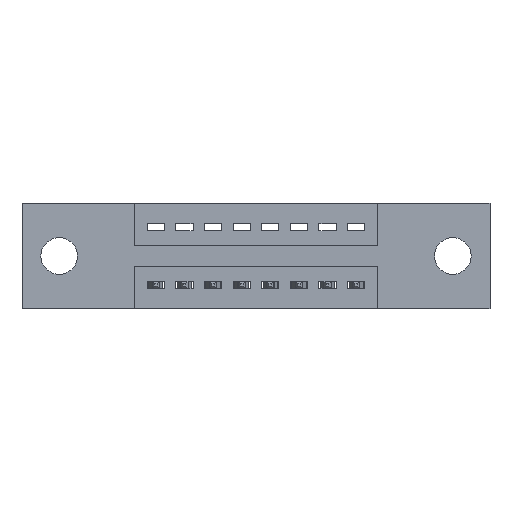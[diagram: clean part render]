
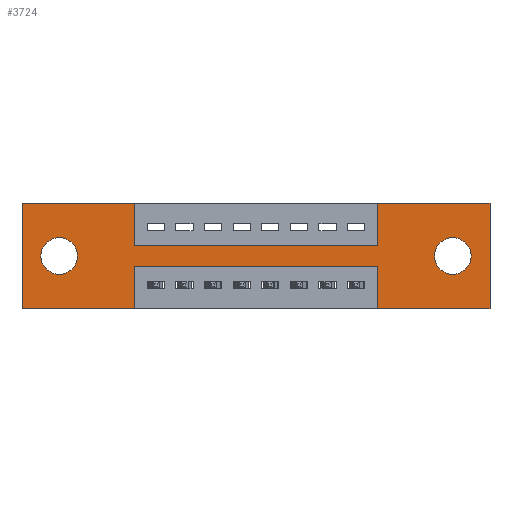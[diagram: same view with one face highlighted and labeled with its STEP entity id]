
A CAD part, front view. The second image highlights one B-rep face of the part: STEP entity #3724.
In plain terms, the highlighted planar face has unit normal (0, -1, 0).
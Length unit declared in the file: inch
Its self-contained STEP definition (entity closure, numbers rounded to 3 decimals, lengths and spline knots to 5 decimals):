
#4 = EDGE_LOOP ( 'NONE', ( #10293, #9271, #5013, #3844, #3061, #8803, #9520, #10448, #2262, #5152, #9273, #4067 ) ) ;
#35 = CIRCLE ( 'NONE', #8697, 0.064 ) ;
#240 = VECTOR ( 'NONE', #6881, 39.37008 ) ;
#347 = CARTESIAN_POINT ( 'NONE',  ( 0.3925, 0., -0.22 ) ) ;
#431 = EDGE_CURVE ( 'NONE', #10010, #1811, #8171, .T. ) ;
#432 = VECTOR ( 'NONE', #6179, 39.37008 ) ;
#490 = DIRECTION ( 'NONE',  ( 0., 0., -1. ) ) ;
#579 = EDGE_LOOP ( 'NONE', ( #4514, #2880 ) ) ;
#806 = CARTESIAN_POINT ( 'NONE',  ( 1.2425, 0., -0.37 ) ) ;
#995 = DIRECTION ( 'NONE',  ( 0., 1., 0. ) ) ;
#1017 = VECTOR ( 'NONE', #2011, 39.37008 ) ;
#1083 = VECTOR ( 'NONE', #9012, 39.37008 ) ;
#1107 = LINE ( 'NONE', #1482, #8126 ) ;
#1212 = VERTEX_POINT ( 'NONE', #10197 ) ;
#1329 = EDGE_CURVE ( 'NONE', #3986, #3708, #7113, .T. ) ;
#1361 = VERTEX_POINT ( 'NONE', #6587 ) ;
#1482 = CARTESIAN_POINT ( 'NONE',  ( 0.3925, 0., -0.37 ) ) ;
#1505 = CARTESIAN_POINT ( 'NONE',  ( 0.3925, 0., 0. ) ) ;
#1555 = CARTESIAN_POINT ( 'NONE',  ( 0.3925, 0., -0.22 ) ) ;
#1620 = CARTESIAN_POINT ( 'NONE',  ( 0., 0., 0. ) ) ;
#1656 = DIRECTION ( 'NONE',  ( 0., 0., 1. ) ) ;
#1811 = VERTEX_POINT ( 'NONE', #9409 ) ;
#1822 = EDGE_CURVE ( 'NONE', #7201, #1212, #8903, .T. ) ;
#1976 = CARTESIAN_POINT ( 'NONE',  ( 1.635, 0., 0. ) ) ;
#2011 = DIRECTION ( 'NONE',  ( 0., 0., -1. ) ) ;
#2190 = VECTOR ( 'NONE', #10179, 39.37008 ) ;
#2245 = CARTESIAN_POINT ( 'NONE',  ( 0.3925, 0., -0.15 ) ) ;
#2262 = ORIENTED_EDGE ( 'NONE', *, *, #7034, .F. ) ;
#2447 = CIRCLE ( 'NONE', #6911, 0.064 ) ;
#2486 = DIRECTION ( 'NONE',  ( 1., 0., 0. ) ) ;
#2880 = ORIENTED_EDGE ( 'NONE', *, *, #4629, .T. ) ;
#3047 = EDGE_CURVE ( 'NONE', #7037, #10362, #4416, .T. ) ;
#3061 = ORIENTED_EDGE ( 'NONE', *, *, #8710, .F. ) ;
#3117 = CARTESIAN_POINT ( 'NONE',  ( 1.635, 0., 0. ) ) ;
#3144 = CARTESIAN_POINT ( 'NONE',  ( 0.3925, 0., -0.37 ) ) ;
#3145 = CARTESIAN_POINT ( 'NONE',  ( 1.505, 0., -0.249 ) ) ;
#3255 = DIRECTION ( 'NONE',  ( -1., 0., 0. ) ) ;
#3258 = VECTOR ( 'NONE', #6969, 39.37008 ) ;
#3501 = FACE_BOUND ( 'NONE', #7701, .T. ) ;
#3543 = CARTESIAN_POINT ( 'NONE',  ( 0.13, 0., -0.185 ) ) ;
#3569 = CARTESIAN_POINT ( 'NONE',  ( 0.13, 0., -0.185 ) ) ;
#3592 = EDGE_CURVE ( 'NONE', #10362, #6763, #8638, .T. ) ;
#3622 = FACE_OUTER_BOUND ( 'NONE', #4, .T. ) ;
#3708 = VERTEX_POINT ( 'NONE', #6121 ) ;
#3709 = CARTESIAN_POINT ( 'NONE',  ( 0., 0., -0.37 ) ) ;
#3724 = ADVANCED_FACE ( 'NONE', ( #4007, #3501, #3622 ), #7742, .T. ) ;
#3844 = ORIENTED_EDGE ( 'NONE', *, *, #5867, .F. ) ;
#3986 = VERTEX_POINT ( 'NONE', #6652 ) ;
#4007 = FACE_BOUND ( 'NONE', #579, .T. ) ;
#4017 = CARTESIAN_POINT ( 'NONE',  ( 0., 0., -0.37 ) ) ;
#4067 = ORIENTED_EDGE ( 'NONE', *, *, #9660, .F. ) ;
#4416 = LINE ( 'NONE', #806, #9458 ) ;
#4480 = DIRECTION ( 'NONE',  ( 0., 1., 0. ) ) ;
#4493 = LINE ( 'NONE', #9876, #10303 ) ;
#4514 = ORIENTED_EDGE ( 'NONE', *, *, #6814, .T. ) ;
#4629 = EDGE_CURVE ( 'NONE', #8817, #1361, #35, .T. ) ;
#4644 = CARTESIAN_POINT ( 'NONE',  ( 0.3925, 0., 0. ) ) ;
#4663 = CARTESIAN_POINT ( 'NONE',  ( 0.13, 0., -0.121 ) ) ;
#4791 = EDGE_CURVE ( 'NONE', #1811, #10010, #5498, .T. ) ;
#4810 = DIRECTION ( 'NONE',  ( -1., 0., 0. ) ) ;
#5013 = ORIENTED_EDGE ( 'NONE', *, *, #3047, .F. ) ;
#5102 = DIRECTION ( 'NONE',  ( 0., 0., -1. ) ) ;
#5148 = LINE ( 'NONE', #4644, #432 ) ;
#5152 = ORIENTED_EDGE ( 'NONE', *, *, #9502, .F. ) ;
#5264 = EDGE_CURVE ( 'NONE', #1212, #7745, #4493, .T. ) ;
#5341 = DIRECTION ( 'NONE',  ( 0., -1., 0. ) ) ;
#5498 = CIRCLE ( 'NONE', #6160, 0.064 ) ;
#5621 = LINE ( 'NONE', #7622, #2190 ) ;
#5657 = VECTOR ( 'NONE', #4810, 39.37008 ) ;
#5718 = EDGE_CURVE ( 'NONE', #9909, #7201, #5621, .T. ) ;
#5867 = EDGE_CURVE ( 'NONE', #8365, #7037, #9819, .T. ) ;
#5886 = CARTESIAN_POINT ( 'NONE',  ( 1.2425, 0., -0.22 ) ) ;
#6008 = ORIENTED_EDGE ( 'NONE', *, *, #431, .T. ) ;
#6051 = DIRECTION ( 'NONE',  ( 0., 0., 1. ) ) ;
#6121 = CARTESIAN_POINT ( 'NONE',  ( 0., 0., 0. ) ) ;
#6160 = AXIS2_PLACEMENT_3D ( 'NONE', #3543, #4480, #6051 ) ;
#6179 = DIRECTION ( 'NONE',  ( 0., 0., -1. ) ) ;
#6543 = CARTESIAN_POINT ( 'NONE',  ( 1.635, 0., -0.37 ) ) ;
#6587 = CARTESIAN_POINT ( 'NONE',  ( 1.505, 0., -0.121 ) ) ;
#6652 = CARTESIAN_POINT ( 'NONE',  ( 0., 0., -0.37 ) ) ;
#6763 = VERTEX_POINT ( 'NONE', #347 ) ;
#6814 = EDGE_CURVE ( 'NONE', #1361, #8817, #2447, .T. ) ;
#6881 = DIRECTION ( 'NONE',  ( 1., 0., 0. ) ) ;
#6893 = CARTESIAN_POINT ( 'NONE',  ( 1.2425, 0., 0. ) ) ;
#6911 = AXIS2_PLACEMENT_3D ( 'NONE', #9196, #995, #5102 ) ;
#6969 = DIRECTION ( 'NONE',  ( 0., 0., 1. ) ) ;
#7034 = EDGE_CURVE ( 'NONE', #9246, #9909, #5148, .T. ) ;
#7037 = VERTEX_POINT ( 'NONE', #7747 ) ;
#7113 = LINE ( 'NONE', #1620, #9728 ) ;
#7178 = DIRECTION ( 'NONE',  ( 0., 0., -1. ) ) ;
#7201 = VERTEX_POINT ( 'NONE', #8494 ) ;
#7617 = DIRECTION ( 'NONE',  ( 0., 0., 1. ) ) ;
#7622 = CARTESIAN_POINT ( 'NONE',  ( 0.3925, 0., -0.15 ) ) ;
#7701 = EDGE_LOOP ( 'NONE', ( #6008, #7990 ) ) ;
#7742 = PLANE ( 'NONE',  #10425 ) ;
#7745 = VERTEX_POINT ( 'NONE', #3117 ) ;
#7747 = CARTESIAN_POINT ( 'NONE',  ( 1.2425, 0., -0.37 ) ) ;
#7762 = DIRECTION ( 'NONE',  ( 0., 0., -1. ) ) ;
#7896 = LINE ( 'NONE', #8159, #8672 ) ;
#7990 = ORIENTED_EDGE ( 'NONE', *, *, #4791, .T. ) ;
#8126 = VECTOR ( 'NONE', #7178, 39.37008 ) ;
#8159 = CARTESIAN_POINT ( 'NONE',  ( 0., 0., -0.37 ) ) ;
#8171 = CIRCLE ( 'NONE', #8312, 0.064 ) ;
#8312 = AXIS2_PLACEMENT_3D ( 'NONE', #3569, #10209, #7617 ) ;
#8365 = VERTEX_POINT ( 'NONE', #6543 ) ;
#8494 = CARTESIAN_POINT ( 'NONE',  ( 1.2425, 0., -0.15 ) ) ;
#8638 = LINE ( 'NONE', #1555, #5657 ) ;
#8672 = VECTOR ( 'NONE', #3255, 39.37008 ) ;
#8697 = AXIS2_PLACEMENT_3D ( 'NONE', #9417, #10206, #7762 ) ;
#8710 = EDGE_CURVE ( 'NONE', #7745, #8365, #10519, .T. ) ;
#8803 = ORIENTED_EDGE ( 'NONE', *, *, #5264, .F. ) ;
#8817 = VERTEX_POINT ( 'NONE', #3145 ) ;
#8903 = LINE ( 'NONE', #6893, #3258 ) ;
#9012 = DIRECTION ( 'NONE',  ( -1., 0., 0. ) ) ;
#9196 = CARTESIAN_POINT ( 'NONE',  ( 1.505, 0., -0.185 ) ) ;
#9246 = VERTEX_POINT ( 'NONE', #1505 ) ;
#9271 = ORIENTED_EDGE ( 'NONE', *, *, #3592, .F. ) ;
#9273 = ORIENTED_EDGE ( 'NONE', *, *, #1329, .F. ) ;
#9337 = VERTEX_POINT ( 'NONE', #3144 ) ;
#9409 = CARTESIAN_POINT ( 'NONE',  ( 0.13, 0., -0.249 ) ) ;
#9417 = CARTESIAN_POINT ( 'NONE',  ( 1.505, 0., -0.185 ) ) ;
#9458 = VECTOR ( 'NONE', #9796, 39.37008 ) ;
#9502 = EDGE_CURVE ( 'NONE', #3708, #9246, #10617, .T. ) ;
#9520 = ORIENTED_EDGE ( 'NONE', *, *, #1822, .F. ) ;
#9660 = EDGE_CURVE ( 'NONE', #9337, #3986, #7896, .T. ) ;
#9728 = VECTOR ( 'NONE', #1656, 39.37008 ) ;
#9789 = CARTESIAN_POINT ( 'NONE',  ( 0., 0., 0. ) ) ;
#9796 = DIRECTION ( 'NONE',  ( 0., 0., 1. ) ) ;
#9819 = LINE ( 'NONE', #4017, #1083 ) ;
#9876 = CARTESIAN_POINT ( 'NONE',  ( 0., 0., 0. ) ) ;
#9909 = VERTEX_POINT ( 'NONE', #2245 ) ;
#10010 = VERTEX_POINT ( 'NONE', #4663 ) ;
#10179 = DIRECTION ( 'NONE',  ( 1., 0., 0. ) ) ;
#10197 = CARTESIAN_POINT ( 'NONE',  ( 1.2425, 0., 0. ) ) ;
#10206 = DIRECTION ( 'NONE',  ( 0., 1., 0. ) ) ;
#10209 = DIRECTION ( 'NONE',  ( 0., 1., 0. ) ) ;
#10293 = ORIENTED_EDGE ( 'NONE', *, *, #10518, .F. ) ;
#10303 = VECTOR ( 'NONE', #2486, 39.37008 ) ;
#10362 = VERTEX_POINT ( 'NONE', #5886 ) ;
#10425 = AXIS2_PLACEMENT_3D ( 'NONE', #3709, #5341, #490 ) ;
#10448 = ORIENTED_EDGE ( 'NONE', *, *, #5718, .F. ) ;
#10518 = EDGE_CURVE ( 'NONE', #6763, #9337, #1107, .T. ) ;
#10519 = LINE ( 'NONE', #1976, #1017 ) ;
#10617 = LINE ( 'NONE', #9789, #240 ) ;
